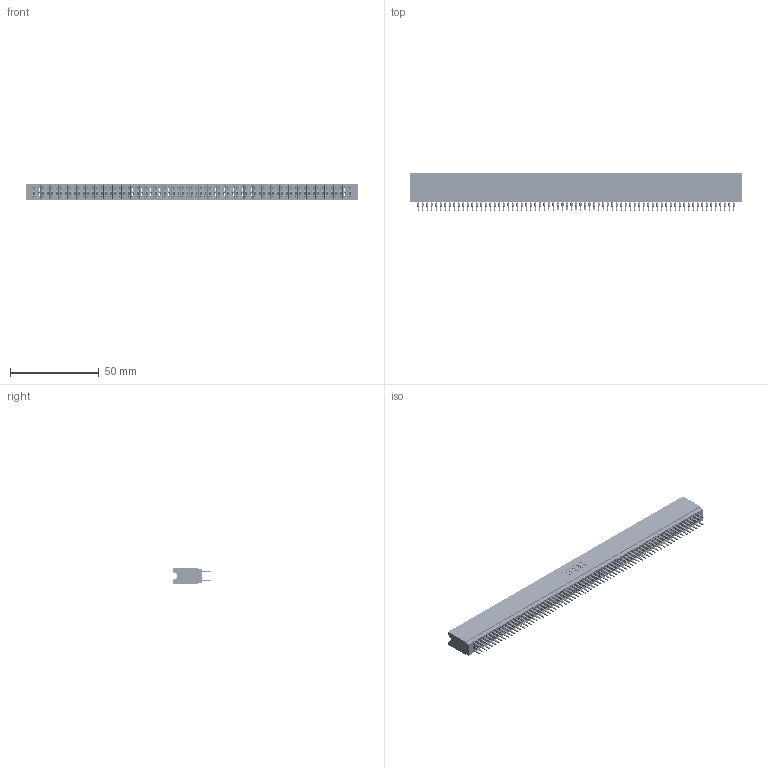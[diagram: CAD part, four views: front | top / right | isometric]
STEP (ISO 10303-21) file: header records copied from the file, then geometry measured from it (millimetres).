
FILE_DESCRIPTION (( 'STEP AP203' ), '1' );
FILE_NAME ('745-142-560-206.STEP', '2026-02-27T04:08:52', ( '' ), ( '' ), 'SwSTEP 2.0', 'SolidWorks 2023', '' );
FILE_SCHEMA (( 'CONFIG_CONTROL_DESIGN' ));
Length unit declared in the file: millimetre
Products named in the file (3): 745 Part_Insulator Option - 06; 745-142-560-206; 745-292-001_560
Assembly tree (143 placements, depth 2):
  745-142-560-206
    745 Part_Insulator Option - 06
    745-292-001_560  x142
Bounding box: 186.94 x 21.22 x 8.89 mm (x, y, z)
Volume: 17163.1 mm3; surface area: 37829.9 mm2
Topology: 143 solids, 143 shells, 14083 faces, 38529 edges, 24454 vertices
Faces by surface type: plane 7298, cylinder 3093, bspline 2840, torus 852
Entity records: 115914 total; most frequent: CARTESIAN_POINT 20600, ORIENTED_EDGE 20094, DIRECTION 17533, EDGE_CURVE 10047, LINE 9431, VECTOR 9431, VERTEX_POINT 6406, AXIS2_PLACEMENT_3D 4051
